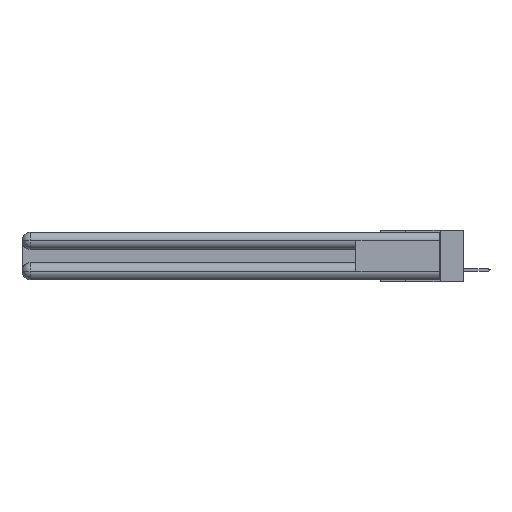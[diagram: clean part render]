
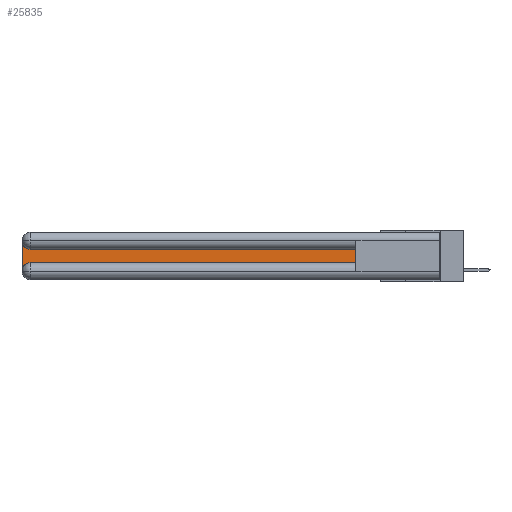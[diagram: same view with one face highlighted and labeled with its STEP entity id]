
A CAD part, left-side view. The second image highlights one B-rep face of the part: STEP entity #25835.
In plain terms, the highlighted planar face has unit normal (-1, 0, 0).
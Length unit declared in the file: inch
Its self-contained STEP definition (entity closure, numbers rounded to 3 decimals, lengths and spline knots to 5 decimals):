
#616 = LINE ( 'NONE', #2347, #17137 ) ;
#1949 = VERTEX_POINT ( 'NONE', #22932 ) ;
#2347 = CARTESIAN_POINT ( 'NONE',  ( 0.075, 0.6, -0.2175 ) ) ;
#3535 = ORIENTED_EDGE ( 'NONE', *, *, #26623, .T. ) ;
#3836 = CARTESIAN_POINT ( 'NONE',  ( 0.075, 0.6, -0.2175 ) ) ;
#3858 = CARTESIAN_POINT ( 'NONE',  ( 0.075, 0.6, -0.1225 ) ) ;
#4282 = PLANE ( 'NONE',  #26251 ) ;
#6170 = EDGE_CURVE ( 'NONE', #30602, #23966, #22778, .T. ) ;
#6305 = EDGE_CURVE ( 'NONE', #12067, #29752, #22743, .T. ) ;
#6474 = ORIENTED_EDGE ( 'NONE', *, *, #6305, .T. ) ;
#7075 = CARTESIAN_POINT ( 'NONE',  ( 0.075, 3., -0.2775 ) ) ;
#7682 = DIRECTION ( 'NONE',  ( 0., 0., -1. ) ) ;
#9131 = ORIENTED_EDGE ( 'NONE', *, *, #25491, .T. ) ;
#11753 = ORIENTED_EDGE ( 'NONE', *, *, #6170, .T. ) ;
#12051 = EDGE_CURVE ( 'NONE', #29752, #1949, #25822, .T. ) ;
#12067 = VERTEX_POINT ( 'NONE', #3836 ) ;
#13596 = CARTESIAN_POINT ( 'NONE',  ( 0.075, 2.94, -0.2775 ) ) ;
#13740 = ORIENTED_EDGE ( 'NONE', *, *, #12051, .T. ) ;
#14002 = DIRECTION ( 'NONE',  ( 0., 0., -1. ) ) ;
#14272 = ORIENTED_EDGE ( 'NONE', *, *, #20030, .T. ) ;
#14757 = EDGE_LOOP ( 'NONE', ( #13740, #14272, #9131, #11753, #3535, #6474 ) ) ;
#14856 = CARTESIAN_POINT ( 'NONE',  ( 0.075, 2.94, -0.2175 ) ) ;
#15575 = CARTESIAN_POINT ( 'NONE',  ( 0.075, 0.6, -0.1225 ) ) ;
#15671 = CARTESIAN_POINT ( 'NONE',  ( 0.075, 3., -0.0625 ) ) ;
#16816 = VECTOR ( 'NONE', #7682, 39.37008 ) ;
#17137 = VECTOR ( 'NONE', #28294, 39.37008 ) ;
#18238 = DIRECTION ( 'NONE',  ( 0., 0., -1. ) ) ;
#18612 = DIRECTION ( 'NONE',  ( 1., 0., 0. ) ) ;
#18713 = DIRECTION ( 'NONE',  ( 0., 0., -1. ) ) ;
#20030 = EDGE_CURVE ( 'NONE', #1949, #24545, #30441, .T. ) ;
#20166 = DIRECTION ( 'NONE',  ( 0., 0., 1. ) ) ;
#21969 = CARTESIAN_POINT ( 'NONE',  ( 0.075, 3., -0.2175 ) ) ;
#22743 = LINE ( 'NONE', #27475, #25334 ) ;
#22778 = CIRCLE ( 'NONE', #28385, 0.06 ) ;
#22932 = CARTESIAN_POINT ( 'NONE',  ( 0.075, 2.94, -0.1225 ) ) ;
#23149 = LINE ( 'NONE', #21969, #16816 ) ;
#23517 = DIRECTION ( 'NONE',  ( 1., 0., 0. ) ) ;
#23632 = AXIS2_PLACEMENT_3D ( 'NONE', #30289, #27648, #18238 ) ;
#23966 = VERTEX_POINT ( 'NONE', #14856 ) ;
#24308 = FACE_OUTER_BOUND ( 'NONE', #14757, .T. ) ;
#24545 = VERTEX_POINT ( 'NONE', #15671 ) ;
#25334 = VECTOR ( 'NONE', #20166, 39.37008 ) ;
#25491 = EDGE_CURVE ( 'NONE', #24545, #30602, #23149, .T. ) ;
#25822 = LINE ( 'NONE', #15575, #30722 ) ;
#25835 = ADVANCED_FACE ( 'NONE', ( #24308 ), #4282, .F. ) ;
#26251 = AXIS2_PLACEMENT_3D ( 'NONE', #28230, #18612, #18713 ) ;
#26623 = EDGE_CURVE ( 'NONE', #23966, #12067, #616, .T. ) ;
#27475 = CARTESIAN_POINT ( 'NONE',  ( 0.075, 0.6, -0.2175 ) ) ;
#27489 = DIRECTION ( 'NONE',  ( 0., 1., 0. ) ) ;
#27648 = DIRECTION ( 'NONE',  ( 1., 0., 0. ) ) ;
#28230 = CARTESIAN_POINT ( 'NONE',  ( 0.075, 3., -0.1225 ) ) ;
#28294 = DIRECTION ( 'NONE',  ( 0., -1., 0. ) ) ;
#28385 = AXIS2_PLACEMENT_3D ( 'NONE', #13596, #23517, #14002 ) ;
#29752 = VERTEX_POINT ( 'NONE', #3858 ) ;
#30289 = CARTESIAN_POINT ( 'NONE',  ( 0.075, 2.94, -0.0625 ) ) ;
#30441 = CIRCLE ( 'NONE', #23632, 0.06 ) ;
#30602 = VERTEX_POINT ( 'NONE', #7075 ) ;
#30722 = VECTOR ( 'NONE', #27489, 39.37008 ) ;
